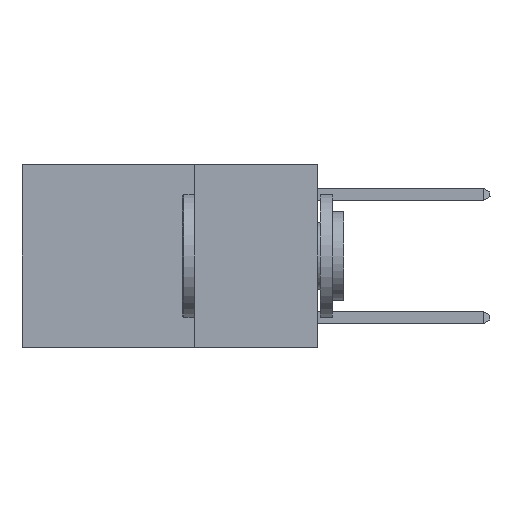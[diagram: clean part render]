
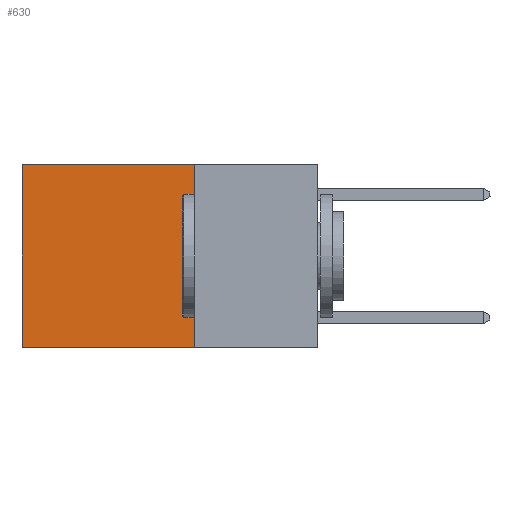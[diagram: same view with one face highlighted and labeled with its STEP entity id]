
A CAD part, left-side view. The second image highlights one B-rep face of the part: STEP entity #630.
In plain terms, the highlighted planar face has unit normal (-1, 0, 0).
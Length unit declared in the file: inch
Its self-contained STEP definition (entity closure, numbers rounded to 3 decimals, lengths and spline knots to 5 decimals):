
#428 = FACE_OUTER_BOUND ( 'NONE', #7026, .T. ) ;
#630 = ADVANCED_FACE ( 'NONE', ( #428 ), #2774, .F. ) ;
#768 = LINE ( 'NONE', #4893, #1069 ) ;
#1056 = LINE ( 'NONE', #7390, #6824 ) ;
#1069 = VECTOR ( 'NONE', #6879, 39.37008 ) ;
#1127 = CARTESIAN_POINT ( 'NONE',  ( 0.2625, 0.25, -0.37 ) ) ;
#1772 = DIRECTION ( 'NONE',  ( 0., 1., 0. ) ) ;
#2774 = PLANE ( 'NONE',  #5094 ) ;
#2862 = CARTESIAN_POINT ( 'NONE',  ( 0.2625, 0.6, 0. ) ) ;
#3105 = CARTESIAN_POINT ( 'NONE',  ( 0.2625, 0.25, 0. ) ) ;
#3165 = EDGE_CURVE ( 'NONE', #8110, #4791, #6848, .T. ) ;
#3394 = DIRECTION ( 'NONE',  ( 1., 0., 0. ) ) ;
#3490 = DIRECTION ( 'NONE',  ( 0., 0., -1. ) ) ;
#4006 = VECTOR ( 'NONE', #1772, 39.37008 ) ;
#4400 = DIRECTION ( 'NONE',  ( 0., 1., 0. ) ) ;
#4538 = EDGE_CURVE ( 'NONE', #4791, #5283, #768, .T. ) ;
#4791 = VERTEX_POINT ( 'NONE', #2862 ) ;
#4893 = CARTESIAN_POINT ( 'NONE',  ( 0.2625, 0.6, 0. ) ) ;
#5094 = AXIS2_PLACEMENT_3D ( 'NONE', #3105, #3394, #3490 ) ;
#5095 = VECTOR ( 'NONE', #4400, 39.37008 ) ;
#5259 = EDGE_CURVE ( 'NONE', #8110, #6394, #1056, .T. ) ;
#5283 = VERTEX_POINT ( 'NONE', #8095 ) ;
#5889 = LINE ( 'NONE', #8065, #4006 ) ;
#6071 = DIRECTION ( 'NONE',  ( 0., 0., -1. ) ) ;
#6394 = VERTEX_POINT ( 'NONE', #1127 ) ;
#6824 = VECTOR ( 'NONE', #6071, 39.37008 ) ;
#6848 = LINE ( 'NONE', #7102, #5095 ) ;
#6879 = DIRECTION ( 'NONE',  ( 0., 0., -1. ) ) ;
#6951 = ORIENTED_EDGE ( 'NONE', *, *, #4538, .T. ) ;
#7026 = EDGE_LOOP ( 'NONE', ( #6951, #7148, #7233, #7260 ) ) ;
#7095 = EDGE_CURVE ( 'NONE', #6394, #5283, #5889, .T. ) ;
#7102 = CARTESIAN_POINT ( 'NONE',  ( 0.2625, 0.25, 0. ) ) ;
#7148 = ORIENTED_EDGE ( 'NONE', *, *, #7095, .F. ) ;
#7233 = ORIENTED_EDGE ( 'NONE', *, *, #5259, .F. ) ;
#7260 = ORIENTED_EDGE ( 'NONE', *, *, #3165, .T. ) ;
#7390 = CARTESIAN_POINT ( 'NONE',  ( 0.2625, 0.25, 0. ) ) ;
#7863 = CARTESIAN_POINT ( 'NONE',  ( 0.2625, 0.25, 0. ) ) ;
#8065 = CARTESIAN_POINT ( 'NONE',  ( 0.2625, 0.25, -0.37 ) ) ;
#8095 = CARTESIAN_POINT ( 'NONE',  ( 0.2625, 0.6, -0.37 ) ) ;
#8110 = VERTEX_POINT ( 'NONE', #7863 ) ;
